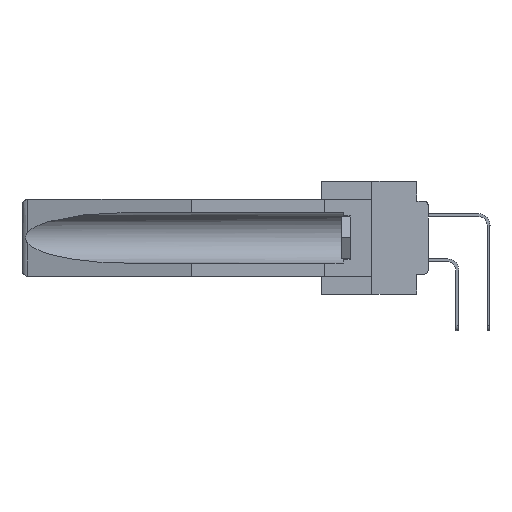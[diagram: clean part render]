
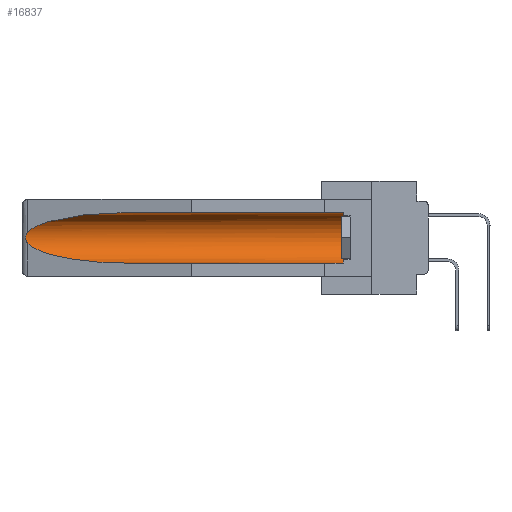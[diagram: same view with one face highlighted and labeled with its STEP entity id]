
A CAD part, left-side view. The second image highlights one B-rep face of the part: STEP entity #16837.
In plain terms, the highlighted cylindrical face has radius 2.857 mm (diameter 5.715 mm), a partial arc.
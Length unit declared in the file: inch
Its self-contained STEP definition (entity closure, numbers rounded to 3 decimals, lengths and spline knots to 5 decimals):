
#1693 = EDGE_LOOP ( 'NONE', ( #29546, #6772, #2900, #23923, #28585, #30569 ) ) ;
#1917 = FACE_OUTER_BOUND ( 'NONE', #1693, .T. ) ;
#2098 = CARTESIAN_POINT ( 'NONE',  ( 0.2673, 1.53269, -0.17917 ) ) ;
#2348 = CARTESIAN_POINT ( 'NONE',  ( 0.26537, 1.52718, -0.19328 ) ) ;
#2688 = CARTESIAN_POINT ( 'NONE',  ( 0.25451, 1.48313, -0.09465 ) ) ;
#2900 = ORIENTED_EDGE ( 'NONE', *, *, #9466, .T. ) ;
#3284 = VECTOR ( 'NONE', #3812, 39.37008 ) ;
#3812 = DIRECTION ( 'NONE',  ( 0., 1., 0. ) ) ;
#6120 = VERTEX_POINT ( 'NONE', #25047 ) ;
#6772 = ORIENTED_EDGE ( 'NONE', *, *, #31723, .T. ) ;
#6988 = CARTESIAN_POINT ( 'NONE',  ( 0.155, 1.07973, -0.284 ) ) ;
#7909 = VERTEX_POINT ( 'NONE', #2348 ) ;
#8922 = CARTESIAN_POINT ( 'NONE',  ( 0.155, -0.30754, -0.284 ) ) ;
#9363 = VERTEX_POINT ( 'NONE', #23336 ) ;
#9466 = EDGE_CURVE ( 'NONE', #7909, #6120, #15081, .T. ) ;
#11689 = EDGE_CURVE ( 'NONE', #17639, #9363, #16267, .T. ) ;
#13994 = CARTESIAN_POINT ( 'NONE',  ( 0.26655, 1.53094, -0.18657 ) ) ;
#14041 = CARTESIAN_POINT ( 'NONE',  ( 0.26537, 1.52718, -0.14972 ) ) ;
#14447 = EDGE_CURVE ( 'NONE', #25142, #17639, #20730, .T. ) ;
#15081 =( BOUNDED_CURVE ( )  B_SPLINE_CURVE ( 3, ( #15712, #21282, #24605, #6988 ),
 .UNSPECIFIED., .F., .F. ) 
 B_SPLINE_CURVE_WITH_KNOTS ( ( 4, 4 ),
 ( 0.1948, 1.5708 ),
 .UNSPECIFIED. ) 
 CURVE ( )  GEOMETRIC_REPRESENTATION_ITEM ( )  RATIONAL_B_SPLINE_CURVE ( ( 1., 0.848, 0.848, 1. ) ) 
 REPRESENTATION_ITEM ( '' )  );
#15712 = CARTESIAN_POINT ( 'NONE',  ( 0.26537, 1.52718, -0.19328 ) ) ;
#16267 =( BOUNDED_CURVE ( )  B_SPLINE_CURVE ( 3, ( #27753, #28126, #2688, #14041 ),
 .UNSPECIFIED., .F., .F. ) 
 B_SPLINE_CURVE_WITH_KNOTS ( ( 4, 4 ),
 ( 4.71239, 6.08839 ),
 .UNSPECIFIED. ) 
 CURVE ( )  GEOMETRIC_REPRESENTATION_ITEM ( )  RATIONAL_B_SPLINE_CURVE ( ( 1., 0.848, 0.848, 1. ) ) 
 REPRESENTATION_ITEM ( '' )  );
#16837 = ADVANCED_FACE ( 'NONE', ( #1917 ), #30129, .F. ) ;
#17068 = CARTESIAN_POINT ( 'NONE',  ( 0.155, -0.30754, -0.059 ) ) ;
#17268 = DIRECTION ( 'NONE',  ( 0., 1., 0. ) ) ;
#17639 = VERTEX_POINT ( 'NONE', #21489 ) ;
#18416 = DIRECTION ( 'NONE',  ( 0., -1., 0. ) ) ;
#18636 = AXIS2_PLACEMENT_3D ( 'NONE', #27879, #30317, #36066 ) ;
#18916 = EDGE_CURVE ( 'NONE', #30381, #25142, #34154, .T. ) ;
#19184 = CARTESIAN_POINT ( 'NONE',  ( 0.2675, 1.53308, -0.16763 ) ) ;
#19540 = CARTESIAN_POINT ( 'NONE',  ( 0.2673, 1.5327, -0.16383 ) ) ;
#19735 = CARTESIAN_POINT ( 'NONE',  ( 0.26537, 1.52718, -0.14972 ) ) ;
#20412 = B_SPLINE_CURVE_WITH_KNOTS ( 'NONE', 3,
 ( #19735, #36071, #30492, #19540, #19184, #30858, #2098, #13994, #31229, #33833 ),
 .UNSPECIFIED., .F., .F.,
 ( 4, 2, 2, 2, 4 ),
 ( 0., 0.00029, 0.00058, 0.00087, 0.00117 ),
 .UNSPECIFIED. ) ;
#20549 = CARTESIAN_POINT ( 'NONE',  ( 0.155, 0.126, -0.284 ) ) ;
#20730 = LINE ( 'NONE', #17068, #3284 ) ;
#21282 = CARTESIAN_POINT ( 'NONE',  ( 0.25451, 1.48313, -0.24835 ) ) ;
#21489 = CARTESIAN_POINT ( 'NONE',  ( 0.155, 1.07973, -0.059 ) ) ;
#21687 = CARTESIAN_POINT ( 'NONE',  ( 0.155, 0.126, -0.059 ) ) ;
#23336 = CARTESIAN_POINT ( 'NONE',  ( 0.26537, 1.52718, -0.14972 ) ) ;
#23621 = CARTESIAN_POINT ( 'NONE',  ( 0.155, 0.126, -0.1715 ) ) ;
#23923 = ORIENTED_EDGE ( 'NONE', *, *, #26823, .F. ) ;
#24605 = CARTESIAN_POINT ( 'NONE',  ( 0.21114, 1.30732, -0.284 ) ) ;
#25047 = CARTESIAN_POINT ( 'NONE',  ( 0.155, 1.07973, -0.284 ) ) ;
#25142 = VERTEX_POINT ( 'NONE', #21687 ) ;
#25987 = LINE ( 'NONE', #8922, #30939 ) ;
#26823 = EDGE_CURVE ( 'NONE', #30381, #6120, #25987, .T. ) ;
#27753 = CARTESIAN_POINT ( 'NONE',  ( 0.155, 1.07973, -0.059 ) ) ;
#27879 = CARTESIAN_POINT ( 'NONE',  ( 0.155, -0.30754, -0.1715 ) ) ;
#28126 = CARTESIAN_POINT ( 'NONE',  ( 0.21114, 1.30732, -0.059 ) ) ;
#28585 = ORIENTED_EDGE ( 'NONE', *, *, #18916, .T. ) ;
#29546 = ORIENTED_EDGE ( 'NONE', *, *, #11689, .T. ) ;
#29550 = DIRECTION ( 'NONE',  ( 0., 0., 1. ) ) ;
#30129 = CYLINDRICAL_SURFACE ( 'NONE', #18636, 0.1125 ) ;
#30317 = DIRECTION ( 'NONE',  ( 0., 1., 0. ) ) ;
#30381 = VERTEX_POINT ( 'NONE', #20549 ) ;
#30492 = CARTESIAN_POINT ( 'NONE',  ( 0.26654, 1.53092, -0.15636 ) ) ;
#30569 = ORIENTED_EDGE ( 'NONE', *, *, #14447, .T. ) ;
#30858 = CARTESIAN_POINT ( 'NONE',  ( 0.2675, 1.53308, -0.17534 ) ) ;
#30939 = VECTOR ( 'NONE', #17268, 39.37008 ) ;
#31229 = CARTESIAN_POINT ( 'NONE',  ( 0.26597, 1.5296, -0.19026 ) ) ;
#31723 = EDGE_CURVE ( 'NONE', #9363, #7909, #20412, .T. ) ;
#33833 = CARTESIAN_POINT ( 'NONE',  ( 0.26537, 1.52718, -0.19328 ) ) ;
#34154 = CIRCLE ( 'NONE', #35933, 0.1125 ) ;
#35933 = AXIS2_PLACEMENT_3D ( 'NONE', #23621, #18416, #29550 ) ;
#36066 = DIRECTION ( 'NONE',  ( 0., 0., 1. ) ) ;
#36071 = CARTESIAN_POINT ( 'NONE',  ( 0.26597, 1.52961, -0.15275 ) ) ;
